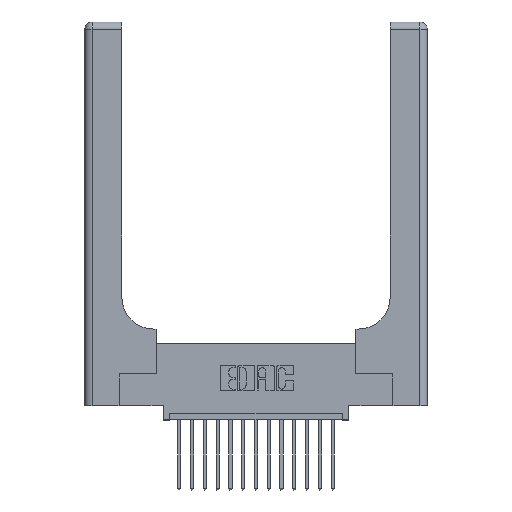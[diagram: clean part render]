
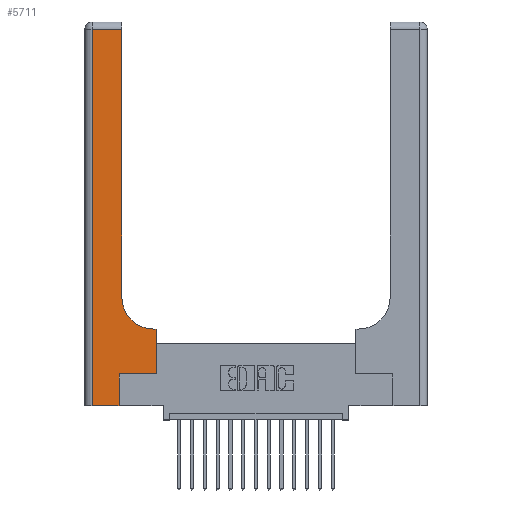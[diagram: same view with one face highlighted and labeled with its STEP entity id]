
A CAD part, top view. The second image highlights one B-rep face of the part: STEP entity #5711.
In plain terms, the highlighted planar face has unit normal (0, 0, 1).
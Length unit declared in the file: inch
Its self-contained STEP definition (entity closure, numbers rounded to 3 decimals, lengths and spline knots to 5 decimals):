
#514 = EDGE_CURVE ( 'NONE', #688, #18473, #7528, .T. ) ;
#688 = VERTEX_POINT ( 'NONE', #14270 ) ;
#865 = DIRECTION ( 'NONE',  ( 0., 1., 0. ) ) ;
#1368 = EDGE_CURVE ( 'NONE', #17458, #8580, #12972, .T. ) ;
#1534 = LINE ( 'NONE', #3477, #16682 ) ;
#1595 = EDGE_CURVE ( 'NONE', #15500, #10447, #10755, .T. ) ;
#1884 = CARTESIAN_POINT ( 'NONE',  ( 0.269, 0., 0.37 ) ) ;
#2099 = VECTOR ( 'NONE', #15538, 39.37008 ) ;
#2295 = DIRECTION ( 'NONE',  ( -1., 0., 0. ) ) ;
#2498 = DIRECTION ( 'NONE',  ( 1., 0., 0. ) ) ;
#2589 = CARTESIAN_POINT ( 'NONE',  ( 0.06, 2.94, 0.37 ) ) ;
#2811 = ORIENTED_EDGE ( 'NONE', *, *, #514, .T. ) ;
#3023 = EDGE_LOOP ( 'NONE', ( #12499, #5609, #17673, #14577, #18483, #14843, #9765, #2811, #16368 ) ) ;
#3362 = CARTESIAN_POINT ( 'NONE',  ( 0.5415, 0.6, 0.37 ) ) ;
#3477 = CARTESIAN_POINT ( 'NONE',  ( 0.269, 0.25, 0.37 ) ) ;
#3904 = CARTESIAN_POINT ( 'NONE',  ( 0., 0., 0.37 ) ) ;
#4900 = VECTOR ( 'NONE', #2498, 39.37008 ) ;
#4938 = DIRECTION ( 'NONE',  ( 1., 0., 0. ) ) ;
#5208 = CARTESIAN_POINT ( 'NONE',  ( 0.2915, 3., 0.37 ) ) ;
#5330 = CARTESIAN_POINT ( 'NONE',  ( 0.5585, 0.25, 0.37 ) ) ;
#5609 = ORIENTED_EDGE ( 'NONE', *, *, #1595, .T. ) ;
#5711 = ADVANCED_FACE ( 'NONE', ( #11219 ), #17273, .F. ) ;
#5931 = VERTEX_POINT ( 'NONE', #13984 ) ;
#6805 = VECTOR ( 'NONE', #16342, 39.37008 ) ;
#7148 = EDGE_CURVE ( 'NONE', #8580, #10498, #1534, .T. ) ;
#7401 = CARTESIAN_POINT ( 'NONE',  ( 0.269, 0., 0.37 ) ) ;
#7491 = VECTOR ( 'NONE', #14282, 39.37008 ) ;
#7528 = LINE ( 'NONE', #16999, #8245 ) ;
#8087 = VECTOR ( 'NONE', #8322, 39.37008 ) ;
#8141 = CARTESIAN_POINT ( 'NONE',  ( 0.06, 0., 0.37 ) ) ;
#8245 = VECTOR ( 'NONE', #2295, 39.37008 ) ;
#8322 = DIRECTION ( 'NONE',  ( 0., 1., 0. ) ) ;
#8580 = VERTEX_POINT ( 'NONE', #16288 ) ;
#8865 = AXIS2_PLACEMENT_3D ( 'NONE', #13520, #9135, #13457 ) ;
#9135 = DIRECTION ( 'NONE',  ( 0., 0., -1. ) ) ;
#9456 = CIRCLE ( 'NONE', #15891, 0.25 ) ;
#9765 = ORIENTED_EDGE ( 'NONE', *, *, #17160, .T. ) ;
#9906 = CARTESIAN_POINT ( 'NONE',  ( 0.2915, 2.94, 0.37 ) ) ;
#10447 = VERTEX_POINT ( 'NONE', #2589 ) ;
#10498 = VERTEX_POINT ( 'NONE', #18886 ) ;
#10611 = LINE ( 'NONE', #5330, #17018 ) ;
#10622 = EDGE_CURVE ( 'NONE', #18473, #5931, #9456, .T. ) ;
#10755 = LINE ( 'NONE', #17224, #6805 ) ;
#10781 = DIRECTION ( 'NONE',  ( 1., 0., 0. ) ) ;
#11219 = FACE_OUTER_BOUND ( 'NONE', #3023, .T. ) ;
#11761 = VERTEX_POINT ( 'NONE', #8141 ) ;
#12499 = ORIENTED_EDGE ( 'NONE', *, *, #16718, .T. ) ;
#12659 = CARTESIAN_POINT ( 'NONE',  ( 0.06, 3., 0.37 ) ) ;
#12972 = LINE ( 'NONE', #1884, #7491 ) ;
#13457 = DIRECTION ( 'NONE',  ( -1., 0., 0. ) ) ;
#13520 = CARTESIAN_POINT ( 'NONE',  ( 0., 3., 0.37 ) ) ;
#13984 = CARTESIAN_POINT ( 'NONE',  ( 0.2915, 0.85, 0.37 ) ) ;
#14270 = CARTESIAN_POINT ( 'NONE',  ( 0.5585, 0.6, 0.37 ) ) ;
#14282 = DIRECTION ( 'NONE',  ( 0., 1., 0. ) ) ;
#14577 = ORIENTED_EDGE ( 'NONE', *, *, #15398, .T. ) ;
#14843 = ORIENTED_EDGE ( 'NONE', *, *, #7148, .T. ) ;
#15117 = DIRECTION ( 'NONE',  ( 0., 0., -1. ) ) ;
#15398 = EDGE_CURVE ( 'NONE', #11761, #17458, #16125, .T. ) ;
#15500 = VERTEX_POINT ( 'NONE', #9906 ) ;
#15538 = DIRECTION ( 'NONE',  ( 0., -1., 0. ) ) ;
#15891 = AXIS2_PLACEMENT_3D ( 'NONE', #16751, #15117, #4938 ) ;
#16125 = LINE ( 'NONE', #3904, #4900 ) ;
#16288 = CARTESIAN_POINT ( 'NONE',  ( 0.269, 0.25, 0.37 ) ) ;
#16342 = DIRECTION ( 'NONE',  ( -1., 0., 0. ) ) ;
#16368 = ORIENTED_EDGE ( 'NONE', *, *, #10622, .T. ) ;
#16532 = LINE ( 'NONE', #12659, #2099 ) ;
#16682 = VECTOR ( 'NONE', #10781, 39.37008 ) ;
#16718 = EDGE_CURVE ( 'NONE', #5931, #15500, #17720, .T. ) ;
#16751 = CARTESIAN_POINT ( 'NONE',  ( 0.5415, 0.85, 0.37 ) ) ;
#16999 = CARTESIAN_POINT ( 'NONE',  ( 0.2915, 0.6, 0.37 ) ) ;
#17018 = VECTOR ( 'NONE', #865, 39.37008 ) ;
#17160 = EDGE_CURVE ( 'NONE', #10498, #688, #10611, .T. ) ;
#17224 = CARTESIAN_POINT ( 'NONE',  ( 0., 2.94, 0.37 ) ) ;
#17228 = EDGE_CURVE ( 'NONE', #10447, #11761, #16532, .T. ) ;
#17273 = PLANE ( 'NONE',  #8865 ) ;
#17458 = VERTEX_POINT ( 'NONE', #7401 ) ;
#17673 = ORIENTED_EDGE ( 'NONE', *, *, #17228, .T. ) ;
#17720 = LINE ( 'NONE', #5208, #8087 ) ;
#18473 = VERTEX_POINT ( 'NONE', #3362 ) ;
#18483 = ORIENTED_EDGE ( 'NONE', *, *, #1368, .T. ) ;
#18886 = CARTESIAN_POINT ( 'NONE',  ( 0.5585, 0.25, 0.37 ) ) ;
